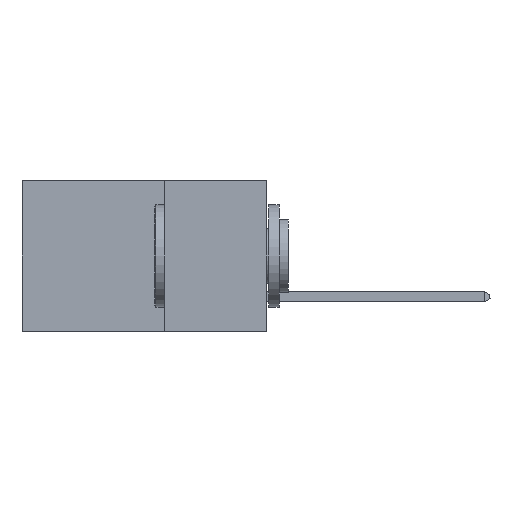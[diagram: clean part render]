
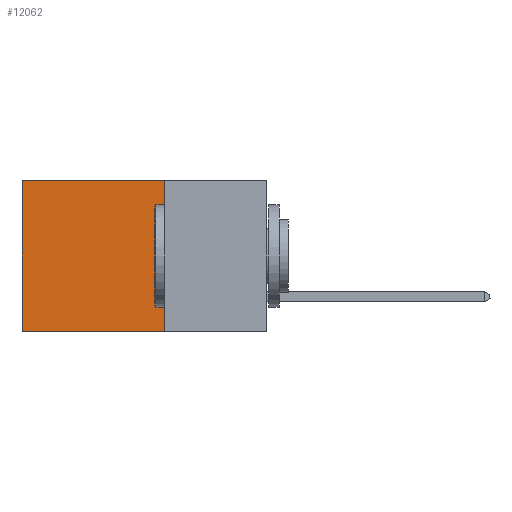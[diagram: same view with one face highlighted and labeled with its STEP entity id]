
A CAD part, left-side view. The second image highlights one B-rep face of the part: STEP entity #12062.
In plain terms, the highlighted planar face has unit normal (-1, 0, 0).
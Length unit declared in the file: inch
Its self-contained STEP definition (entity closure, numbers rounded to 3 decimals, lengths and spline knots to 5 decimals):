
#1249 = DIRECTION ( 'NONE',  ( 0., 0., -1. ) ) ;
#1282 = VERTEX_POINT ( 'NONE', #34669 ) ;
#1547 = EDGE_CURVE ( 'NONE', #6747, #8769, #3206, .T. ) ;
#1985 = VECTOR ( 'NONE', #8425, 39.37008 ) ;
#2941 = ORIENTED_EDGE ( 'NONE', *, *, #7463, .F. ) ;
#3206 = LINE ( 'NONE', #22824, #36777 ) ;
#3608 = LINE ( 'NONE', #41892, #32217 ) ;
#5307 = AXIS2_PLACEMENT_3D ( 'NONE', #12597, #15734, #15589 ) ;
#6747 = VERTEX_POINT ( 'NONE', #39868 ) ;
#7374 = CARTESIAN_POINT ( 'NONE',  ( 0.2875, 0.25, 0. ) ) ;
#7463 = EDGE_CURVE ( 'NONE', #33504, #6747, #3608, .T. ) ;
#8425 = DIRECTION ( 'NONE',  ( 0., 1., 0. ) ) ;
#8769 = VERTEX_POINT ( 'NONE', #37583 ) ;
#9334 = PLANE ( 'NONE',  #5307 ) ;
#12062 = ADVANCED_FACE ( 'NONE', ( #36329 ), #9334, .F. ) ;
#12597 = CARTESIAN_POINT ( 'NONE',  ( 0.2875, 0.25, 0. ) ) ;
#12764 = DIRECTION ( 'NONE',  ( 0., 0., -1. ) ) ;
#12982 = EDGE_LOOP ( 'NONE', ( #23059, #35514, #2941, #28737 ) ) ;
#14129 = CARTESIAN_POINT ( 'NONE',  ( 0.2875, 0.6, 0. ) ) ;
#15589 = DIRECTION ( 'NONE',  ( 0., 0., -1. ) ) ;
#15734 = DIRECTION ( 'NONE',  ( 1., 0., 0. ) ) ;
#17849 = CARTESIAN_POINT ( 'NONE',  ( 0.2875, 0.25, 0. ) ) ;
#20260 = EDGE_CURVE ( 'NONE', #33504, #1282, #28585, .T. ) ;
#20580 = EDGE_CURVE ( 'NONE', #1282, #8769, #33600, .T. ) ;
#22824 = CARTESIAN_POINT ( 'NONE',  ( 0.2875, 0.25, -0.37 ) ) ;
#22900 = VECTOR ( 'NONE', #1249, 39.37008 ) ;
#23059 = ORIENTED_EDGE ( 'NONE', *, *, #20580, .T. ) ;
#28585 = LINE ( 'NONE', #17849, #1985 ) ;
#28737 = ORIENTED_EDGE ( 'NONE', *, *, #20260, .T. ) ;
#31126 = DIRECTION ( 'NONE',  ( 0., 1., 0. ) ) ;
#32217 = VECTOR ( 'NONE', #12764, 39.37008 ) ;
#33504 = VERTEX_POINT ( 'NONE', #7374 ) ;
#33600 = LINE ( 'NONE', #14129, #22900 ) ;
#34669 = CARTESIAN_POINT ( 'NONE',  ( 0.2875, 0.6, 0. ) ) ;
#35514 = ORIENTED_EDGE ( 'NONE', *, *, #1547, .F. ) ;
#36329 = FACE_OUTER_BOUND ( 'NONE', #12982, .T. ) ;
#36777 = VECTOR ( 'NONE', #31126, 39.37008 ) ;
#37583 = CARTESIAN_POINT ( 'NONE',  ( 0.2875, 0.6, -0.37 ) ) ;
#39868 = CARTESIAN_POINT ( 'NONE',  ( 0.2875, 0.25, -0.37 ) ) ;
#41892 = CARTESIAN_POINT ( 'NONE',  ( 0.2875, 0.25, 0. ) ) ;
